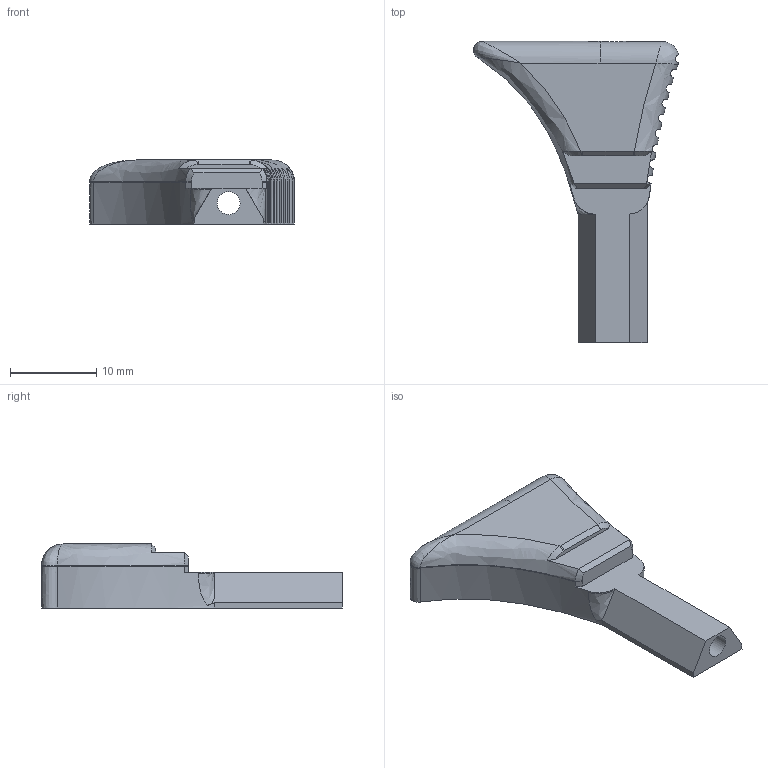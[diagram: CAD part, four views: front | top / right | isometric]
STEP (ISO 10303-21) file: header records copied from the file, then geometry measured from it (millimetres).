
FILE_DESCRIPTION(/* description */ (''),/* implementation_level */ '2;1');
FILE_NAME(/* name */ 'charging handle.step',/* time_stamp */ '2021-09-02T19:33:30-05:00',/* author */ (''),/* organization */ (''),/* preprocessor_version */ 'ST-DEVELOPER v18.1',/* originating_system */ 'Autodesk Translation Framework v10.10.0.1391',/* authorisation */ '');
FILE_SCHEMA (('AUTOMOTIVE_DESIGN { 1 0 10303 214 3 1 1 }'));
Length unit declared in the file: millimetre
Products named in the file (1): latest charging handle (1)
Bounding box: 23.74 x 34.86 x 7.42 mm (x, y, z)
Volume: 2063.7 mm3; surface area: 1669.2 mm2
Topology: 1 solids, 1 shells, 78 faces, 219 edges, 141 vertices
Faces by surface type: bspline 46, plane 19, cylinder 13
Full cylindrical faces by diameter (mm): 2.65 x1
Entity records: 4412 total; most frequent: CARTESIAN_POINT 2797, ORIENTED_EDGE 434, EDGE_CURVE 217, DIRECTION 159, B_SPLINE_CURVE_WITH_KNOTS 146, VERTEX_POINT 141, EDGE_LOOP 80, FACE_OUTER_BOUND 78
